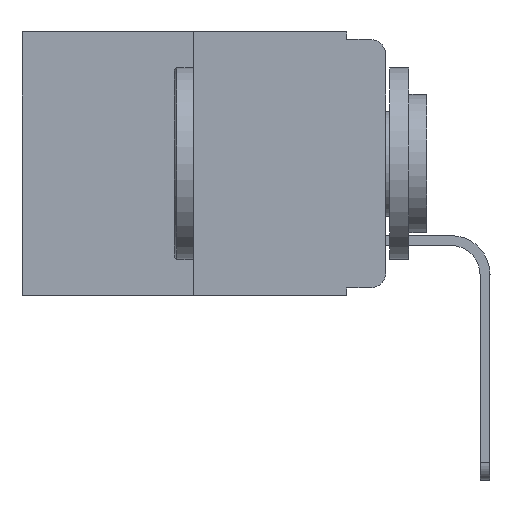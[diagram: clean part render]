
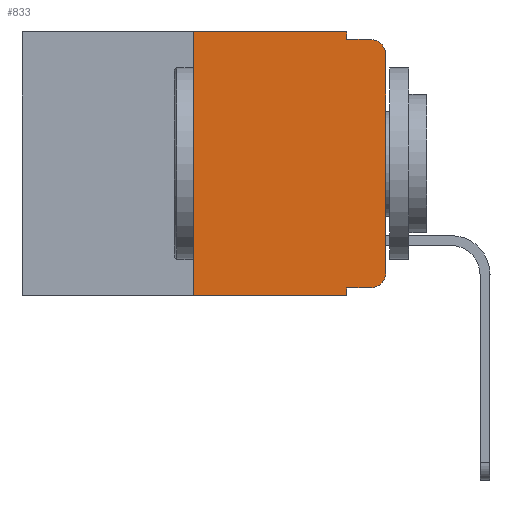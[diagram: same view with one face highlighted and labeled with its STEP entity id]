
A CAD part, left-side view. The second image highlights one B-rep face of the part: STEP entity #833.
In plain terms, the highlighted planar face has unit normal (-1, 0, 0).
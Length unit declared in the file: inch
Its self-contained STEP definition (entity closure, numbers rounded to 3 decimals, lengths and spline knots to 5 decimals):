
#180 = DIRECTION ( 'NONE',  ( 0., 0., -1. ) ) ;
#420 = EDGE_CURVE ( 'NONE', #3287, #3124, #7080, .T. ) ;
#793 = CARTESIAN_POINT ( 'NONE',  ( 0., 0.02, -0.333 ) ) ;
#825 = ORIENTED_EDGE ( 'NONE', *, *, #420, .T. ) ;
#833 = ADVANCED_FACE ( 'NONE', ( #8594 ), #7751, .F. ) ;
#852 = CARTESIAN_POINT ( 'NONE',  ( 0., 0.051, 0. ) ) ;
#898 = DIRECTION ( 'NONE',  ( 0., 0., -1. ) ) ;
#975 = CARTESIAN_POINT ( 'NONE',  ( 0., 0.051, -0.333 ) ) ;
#997 = VERTEX_POINT ( 'NONE', #793 ) ;
#1029 = DIRECTION ( 'NONE',  ( 0., 0., 1. ) ) ;
#1141 = CARTESIAN_POINT ( 'NONE',  ( 0., 0.02, -0.01 ) ) ;
#1189 = AXIS2_PLACEMENT_3D ( 'NONE', #1648, #6566, #15177 ) ;
#1450 = DIRECTION ( 'NONE',  ( 0., -1., 0. ) ) ;
#1537 = AXIS2_PLACEMENT_3D ( 'NONE', #13167, #5738, #898 ) ;
#1600 = ORIENTED_EDGE ( 'NONE', *, *, #12759, .F. ) ;
#1639 = VERTEX_POINT ( 'NONE', #11858 ) ;
#1648 = CARTESIAN_POINT ( 'NONE',  ( 0., 0.473, 0. ) ) ;
#1924 = DIRECTION ( 'NONE',  ( 0., 0., -1. ) ) ;
#2547 = ORIENTED_EDGE ( 'NONE', *, *, #4224, .T. ) ;
#2565 = CIRCLE ( 'NONE', #1537, 0.02 ) ;
#3075 = EDGE_CURVE ( 'NONE', #12238, #3908, #12206, .T. ) ;
#3076 = VERTEX_POINT ( 'NONE', #3944 ) ;
#3124 = VERTEX_POINT ( 'NONE', #7684 ) ;
#3220 = CARTESIAN_POINT ( 'NONE',  ( 0., 0., 0. ) ) ;
#3287 = VERTEX_POINT ( 'NONE', #10626 ) ;
#3908 = VERTEX_POINT ( 'NONE', #1141 ) ;
#3944 = CARTESIAN_POINT ( 'NONE',  ( 0., 0.25, 0. ) ) ;
#4224 = EDGE_CURVE ( 'NONE', #4438, #1639, #5847, .T. ) ;
#4230 = DIRECTION ( 'NONE',  ( 0., -1., 0. ) ) ;
#4438 = VERTEX_POINT ( 'NONE', #14469 ) ;
#4571 = LINE ( 'NONE', #7491, #10691 ) ;
#5028 = CARTESIAN_POINT ( 'NONE',  ( 0., 0.051, -0.01 ) ) ;
#5593 = LINE ( 'NONE', #852, #10941 ) ;
#5738 = DIRECTION ( 'NONE',  ( -1., 0., 0. ) ) ;
#5751 = ORIENTED_EDGE ( 'NONE', *, *, #3075, .F. ) ;
#5760 = DIRECTION ( 'NONE',  ( 0., -1., 0. ) ) ;
#5847 = LINE ( 'NONE', #14201, #9461 ) ;
#6021 = VERTEX_POINT ( 'NONE', #7904 ) ;
#6252 = VECTOR ( 'NONE', #15044, 39.37008 ) ;
#6566 = DIRECTION ( 'NONE',  ( 1., 0., 0. ) ) ;
#7080 = LINE ( 'NONE', #3220, #9195 ) ;
#7366 = ORIENTED_EDGE ( 'NONE', *, *, #13166, .T. ) ;
#7454 = EDGE_CURVE ( 'NONE', #997, #3287, #2565, .T. ) ;
#7491 = CARTESIAN_POINT ( 'NONE',  ( 0., 0.051, 0. ) ) ;
#7684 = CARTESIAN_POINT ( 'NONE',  ( 0., 0., -0.03 ) ) ;
#7751 = PLANE ( 'NONE',  #1189 ) ;
#7805 = VECTOR ( 'NONE', #1450, 39.37008 ) ;
#7904 = CARTESIAN_POINT ( 'NONE',  ( 0., 0.051, 0. ) ) ;
#8571 = VECTOR ( 'NONE', #5760, 39.37008 ) ;
#8594 = FACE_OUTER_BOUND ( 'NONE', #9710, .T. ) ;
#8657 = CARTESIAN_POINT ( 'NONE',  ( 0., 0.02, -0.03 ) ) ;
#9195 = VECTOR ( 'NONE', #1029, 39.37008 ) ;
#9240 = EDGE_CURVE ( 'NONE', #6021, #12238, #5593, .T. ) ;
#9461 = VECTOR ( 'NONE', #4230, 39.37008 ) ;
#9710 = EDGE_LOOP ( 'NONE', ( #825, #7366, #5751, #15246, #14185, #1600, #2547, #11283, #10574, #14129 ) ) ;
#10114 = CARTESIAN_POINT ( 'NONE',  ( 0., 0.25, 0. ) ) ;
#10574 = ORIENTED_EDGE ( 'NONE', *, *, #11433, .T. ) ;
#10626 = CARTESIAN_POINT ( 'NONE',  ( 0., 0., -0.313 ) ) ;
#10691 = VECTOR ( 'NONE', #180, 39.37008 ) ;
#10941 = VECTOR ( 'NONE', #1924, 39.37008 ) ;
#11073 = LINE ( 'NONE', #14926, #7805 ) ;
#11174 = EDGE_CURVE ( 'NONE', #3076, #6021, #11073, .T. ) ;
#11283 = ORIENTED_EDGE ( 'NONE', *, *, #12725, .F. ) ;
#11433 = EDGE_CURVE ( 'NONE', #15329, #997, #15707, .T. ) ;
#11657 = CIRCLE ( 'NONE', #12196, 0.02 ) ;
#11858 = CARTESIAN_POINT ( 'NONE',  ( 0., 0.051, -0.343 ) ) ;
#12196 = AXIS2_PLACEMENT_3D ( 'NONE', #8657, #12303, #13383 ) ;
#12206 = LINE ( 'NONE', #13655, #6252 ) ;
#12238 = VERTEX_POINT ( 'NONE', #5028 ) ;
#12240 = LINE ( 'NONE', #10114, #14360 ) ;
#12303 = DIRECTION ( 'NONE',  ( -1., 0., 0. ) ) ;
#12725 = EDGE_CURVE ( 'NONE', #15329, #1639, #4571, .T. ) ;
#12759 = EDGE_CURVE ( 'NONE', #4438, #3076, #12240, .T. ) ;
#13166 = EDGE_CURVE ( 'NONE', #3124, #3908, #11657, .T. ) ;
#13167 = CARTESIAN_POINT ( 'NONE',  ( 0., 0.02, -0.313 ) ) ;
#13383 = DIRECTION ( 'NONE',  ( 0., 0., -1. ) ) ;
#13655 = CARTESIAN_POINT ( 'NONE',  ( 0., 0.051, -0.01 ) ) ;
#13984 = DIRECTION ( 'NONE',  ( 0., 0., 1. ) ) ;
#14129 = ORIENTED_EDGE ( 'NONE', *, *, #7454, .T. ) ;
#14185 = ORIENTED_EDGE ( 'NONE', *, *, #11174, .F. ) ;
#14201 = CARTESIAN_POINT ( 'NONE',  ( 0., 0.473, -0.343 ) ) ;
#14247 = CARTESIAN_POINT ( 'NONE',  ( 0., 0.051, -0.333 ) ) ;
#14360 = VECTOR ( 'NONE', #13984, 39.37008 ) ;
#14469 = CARTESIAN_POINT ( 'NONE',  ( 0., 0.25, -0.343 ) ) ;
#14926 = CARTESIAN_POINT ( 'NONE',  ( 0., 0.473, 0. ) ) ;
#15044 = DIRECTION ( 'NONE',  ( 0., -1., 0. ) ) ;
#15177 = DIRECTION ( 'NONE',  ( 0., 0., -1. ) ) ;
#15246 = ORIENTED_EDGE ( 'NONE', *, *, #9240, .F. ) ;
#15329 = VERTEX_POINT ( 'NONE', #14247 ) ;
#15707 = LINE ( 'NONE', #975, #8571 ) ;
